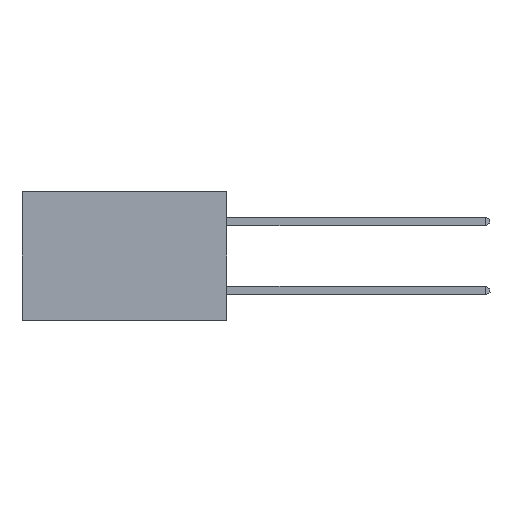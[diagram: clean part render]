
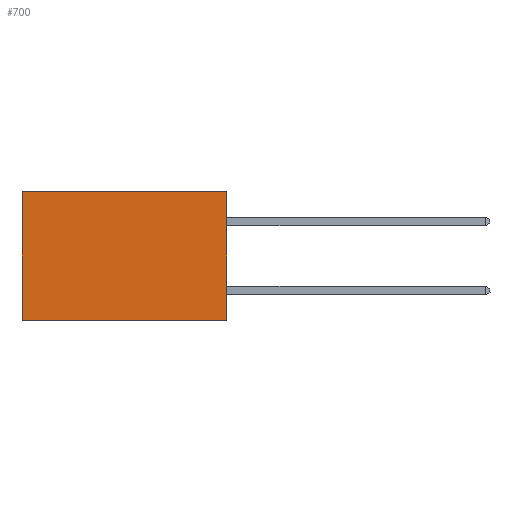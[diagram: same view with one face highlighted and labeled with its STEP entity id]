
A CAD part, left-side view. The second image highlights one B-rep face of the part: STEP entity #700.
In plain terms, the highlighted planar face has unit normal (-1, 0, 0).
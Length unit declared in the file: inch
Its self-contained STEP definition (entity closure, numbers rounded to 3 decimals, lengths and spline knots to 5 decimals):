
#26 = ORIENTED_EDGE ( 'NONE', *, *, #5668, .T. ) ;
#110 = LINE ( 'NONE', #9233, #8180 ) ;
#123 = DIRECTION ( 'NONE',  ( 0., 0., -1. ) ) ;
#253 = EDGE_CURVE ( 'NONE', #1305, #8914, #110, .T. ) ;
#700 = ADVANCED_FACE ( 'NONE', ( #5825 ), #7533, .F. ) ;
#1046 = AXIS2_PLACEMENT_3D ( 'NONE', #2787, #2828, #3846 ) ;
#1088 = VERTEX_POINT ( 'NONE', #8907 ) ;
#1249 = ORIENTED_EDGE ( 'NONE', *, *, #4521, .T. ) ;
#1305 = VERTEX_POINT ( 'NONE', #1780 ) ;
#1548 = VECTOR ( 'NONE', #8034, 39.37008 ) ;
#1552 = DIRECTION ( 'NONE',  ( 0., 1., 0. ) ) ;
#1598 = CARTESIAN_POINT ( 'NONE',  ( 0.277, 0., 0. ) ) ;
#1780 = CARTESIAN_POINT ( 'NONE',  ( 0.277, 0., 0. ) ) ;
#2106 = EDGE_LOOP ( 'NONE', ( #1249, #3608, #5637, #26 ) ) ;
#2445 = EDGE_CURVE ( 'NONE', #8914, #5046, #9119, .T. ) ;
#2486 = DIRECTION ( 'NONE',  ( 0., 0., -1. ) ) ;
#2781 = CARTESIAN_POINT ( 'NONE',  ( 0.277, 0.59, -0.37 ) ) ;
#2787 = CARTESIAN_POINT ( 'NONE',  ( 0.277, 0., -0.37 ) ) ;
#2828 = DIRECTION ( 'NONE',  ( 1., 0., 0. ) ) ;
#3608 = ORIENTED_EDGE ( 'NONE', *, *, #2445, .F. ) ;
#3620 = VECTOR ( 'NONE', #2486, 39.37008 ) ;
#3846 = DIRECTION ( 'NONE',  ( 0., 0., -1. ) ) ;
#4521 = EDGE_CURVE ( 'NONE', #1088, #5046, #9488, .T. ) ;
#4661 = LINE ( 'NONE', #1598, #5862 ) ;
#5046 = VERTEX_POINT ( 'NONE', #6595 ) ;
#5637 = ORIENTED_EDGE ( 'NONE', *, *, #253, .F. ) ;
#5668 = EDGE_CURVE ( 'NONE', #1305, #1088, #4661, .T. ) ;
#5825 = FACE_OUTER_BOUND ( 'NONE', #2106, .T. ) ;
#5862 = VECTOR ( 'NONE', #1552, 39.37008 ) ;
#6595 = CARTESIAN_POINT ( 'NONE',  ( 0.277, 0.59, -0.37 ) ) ;
#7533 = PLANE ( 'NONE',  #1046 ) ;
#7988 = CARTESIAN_POINT ( 'NONE',  ( 0.277, 0., -0.37 ) ) ;
#8034 = DIRECTION ( 'NONE',  ( 0., 1., 0. ) ) ;
#8180 = VECTOR ( 'NONE', #123, 39.37008 ) ;
#8907 = CARTESIAN_POINT ( 'NONE',  ( 0.277, 0.59, 0. ) ) ;
#8914 = VERTEX_POINT ( 'NONE', #9532 ) ;
#9119 = LINE ( 'NONE', #7988, #1548 ) ;
#9233 = CARTESIAN_POINT ( 'NONE',  ( 0.277, 0., -0.37 ) ) ;
#9488 = LINE ( 'NONE', #2781, #3620 ) ;
#9532 = CARTESIAN_POINT ( 'NONE',  ( 0.277, 0., -0.37 ) ) ;
